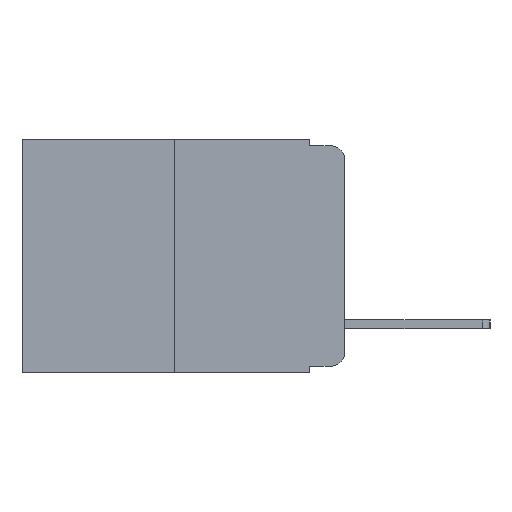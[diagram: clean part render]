
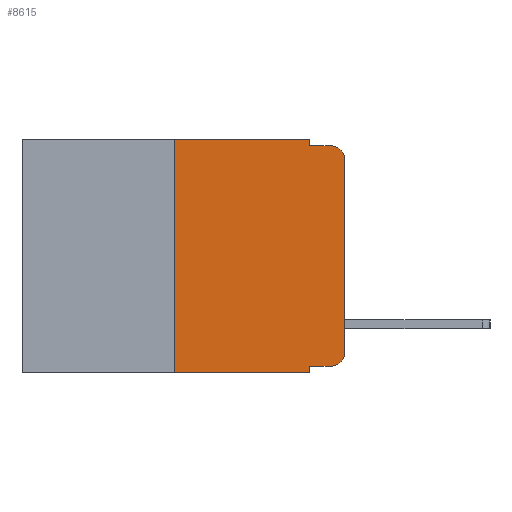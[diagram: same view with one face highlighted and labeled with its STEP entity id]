
A CAD part, left-side view. The second image highlights one B-rep face of the part: STEP entity #8615.
In plain terms, the highlighted planar face has unit normal (-1, 0, 0).
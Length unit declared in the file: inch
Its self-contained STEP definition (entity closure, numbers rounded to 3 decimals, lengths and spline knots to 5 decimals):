
#143 = FACE_OUTER_BOUND ( 'NONE', #7279, .T. ) ;
#237 = LINE ( 'NONE', #8047, #12402 ) ;
#459 = ORIENTED_EDGE ( 'NONE', *, *, #11915, .T. ) ;
#622 = CARTESIAN_POINT ( 'NONE',  ( 0., 0., -0.03 ) ) ;
#645 = PLANE ( 'NONE',  #2791 ) ;
#674 = ORIENTED_EDGE ( 'NONE', *, *, #12415, .T. ) ;
#821 = VECTOR ( 'NONE', #10563, 39.37008 ) ;
#980 = CIRCLE ( 'NONE', #7536, 0.02 ) ;
#990 = CARTESIAN_POINT ( 'NONE',  ( 0., 0.02, -0.03 ) ) ;
#1172 = CARTESIAN_POINT ( 'NONE',  ( 0., 0.25, 0. ) ) ;
#1273 = CARTESIAN_POINT ( 'NONE',  ( 0., 0.25, -0.343 ) ) ;
#1564 = VECTOR ( 'NONE', #3622, 39.37008 ) ;
#1577 = DIRECTION ( 'NONE',  ( 0., -1., 0. ) ) ;
#1594 = DIRECTION ( 'NONE',  ( 0., 0., -1. ) ) ;
#1650 = CARTESIAN_POINT ( 'NONE',  ( 0., 0.473, -0.343 ) ) ;
#1664 = VERTEX_POINT ( 'NONE', #1273 ) ;
#1936 = DIRECTION ( 'NONE',  ( 0., 0., -1. ) ) ;
#2309 = AXIS2_PLACEMENT_3D ( 'NONE', #3073, #9884, #4076 ) ;
#2432 = CARTESIAN_POINT ( 'NONE',  ( 0., 0.25, 0. ) ) ;
#2791 = AXIS2_PLACEMENT_3D ( 'NONE', #11223, #7389, #1594 ) ;
#2829 = VERTEX_POINT ( 'NONE', #8810 ) ;
#3045 = VECTOR ( 'NONE', #7934, 39.37008 ) ;
#3073 = CARTESIAN_POINT ( 'NONE',  ( 0., 0.02, -0.313 ) ) ;
#3076 = CARTESIAN_POINT ( 'NONE',  ( 0., 0., -0.313 ) ) ;
#3243 = EDGE_CURVE ( 'NONE', #12396, #8947, #980, .T. ) ;
#3322 = VECTOR ( 'NONE', #12444, 39.37008 ) ;
#3503 = CARTESIAN_POINT ( 'NONE',  ( 0., 0.051, -0.333 ) ) ;
#3551 = ORIENTED_EDGE ( 'NONE', *, *, #3653, .T. ) ;
#3622 = DIRECTION ( 'NONE',  ( 0., -1., 0. ) ) ;
#3653 = EDGE_CURVE ( 'NONE', #1664, #4661, #4457, .T. ) ;
#3947 = EDGE_CURVE ( 'NONE', #7925, #6077, #5672, .T. ) ;
#3960 = VECTOR ( 'NONE', #7903, 39.37008 ) ;
#4023 = EDGE_CURVE ( 'NONE', #6077, #8228, #237, .T. ) ;
#4049 = CARTESIAN_POINT ( 'NONE',  ( 0., 0.051, 0. ) ) ;
#4076 = DIRECTION ( 'NONE',  ( 0., 0., -1. ) ) ;
#4186 = DIRECTION ( 'NONE',  ( 0., 0., -1. ) ) ;
#4278 = ORIENTED_EDGE ( 'NONE', *, *, #11878, .F. ) ;
#4457 = LINE ( 'NONE', #1650, #1564 ) ;
#4657 = EDGE_CURVE ( 'NONE', #4885, #12396, #11209, .T. ) ;
#4661 = VERTEX_POINT ( 'NONE', #4732 ) ;
#4708 = VERTEX_POINT ( 'NONE', #4804 ) ;
#4732 = CARTESIAN_POINT ( 'NONE',  ( 0., 0.051, -0.343 ) ) ;
#4804 = CARTESIAN_POINT ( 'NONE',  ( 0., 0.02, -0.333 ) ) ;
#4885 = VERTEX_POINT ( 'NONE', #3076 ) ;
#4922 = ORIENTED_EDGE ( 'NONE', *, *, #11951, .F. ) ;
#5312 = ORIENTED_EDGE ( 'NONE', *, *, #4657, .T. ) ;
#5422 = ORIENTED_EDGE ( 'NONE', *, *, #3243, .T. ) ;
#5672 = LINE ( 'NONE', #8899, #3045 ) ;
#5780 = CARTESIAN_POINT ( 'NONE',  ( 0., 0.051, -0.01 ) ) ;
#5969 = LINE ( 'NONE', #1172, #3322 ) ;
#6006 = LINE ( 'NONE', #5780, #821 ) ;
#6077 = VERTEX_POINT ( 'NONE', #4049 ) ;
#6549 = LINE ( 'NONE', #11723, #3960 ) ;
#7279 = EDGE_LOOP ( 'NONE', ( #5312, #5422, #11512, #7449, #9998, #4922, #3551, #4278, #674, #459 ) ) ;
#7389 = DIRECTION ( 'NONE',  ( 1., 0., 0. ) ) ;
#7449 = ORIENTED_EDGE ( 'NONE', *, *, #4023, .F. ) ;
#7536 = AXIS2_PLACEMENT_3D ( 'NONE', #990, #7769, #1936 ) ;
#7769 = DIRECTION ( 'NONE',  ( -1., 0., 0. ) ) ;
#7903 = DIRECTION ( 'NONE',  ( 0., 0., -1. ) ) ;
#7925 = VERTEX_POINT ( 'NONE', #2432 ) ;
#7934 = DIRECTION ( 'NONE',  ( 0., -1., 0. ) ) ;
#8047 = CARTESIAN_POINT ( 'NONE',  ( 0., 0.051, 0. ) ) ;
#8228 = VERTEX_POINT ( 'NONE', #9648 ) ;
#8615 = ADVANCED_FACE ( 'NONE', ( #143 ), #645, .F. ) ;
#8810 = CARTESIAN_POINT ( 'NONE',  ( 0., 0.051, -0.333 ) ) ;
#8823 = CIRCLE ( 'NONE', #2309, 0.02 ) ;
#8899 = CARTESIAN_POINT ( 'NONE',  ( 0., 0.473, 0. ) ) ;
#8947 = VERTEX_POINT ( 'NONE', #9805 ) ;
#9648 = CARTESIAN_POINT ( 'NONE',  ( 0., 0.051, -0.01 ) ) ;
#9805 = CARTESIAN_POINT ( 'NONE',  ( 0., 0.02, -0.01 ) ) ;
#9884 = DIRECTION ( 'NONE',  ( -1., 0., 0. ) ) ;
#9998 = ORIENTED_EDGE ( 'NONE', *, *, #3947, .F. ) ;
#10033 = VECTOR ( 'NONE', #1577, 39.37008 ) ;
#10506 = CARTESIAN_POINT ( 'NONE',  ( 0., 0., 0. ) ) ;
#10563 = DIRECTION ( 'NONE',  ( 0., -1., 0. ) ) ;
#10576 = EDGE_CURVE ( 'NONE', #8228, #8947, #6006, .T. ) ;
#10922 = VECTOR ( 'NONE', #11462, 39.37008 ) ;
#11209 = LINE ( 'NONE', #10506, #10922 ) ;
#11214 = LINE ( 'NONE', #3503, #10033 ) ;
#11223 = CARTESIAN_POINT ( 'NONE',  ( 0., 0.473, 0. ) ) ;
#11462 = DIRECTION ( 'NONE',  ( 0., 0., 1. ) ) ;
#11512 = ORIENTED_EDGE ( 'NONE', *, *, #10576, .F. ) ;
#11723 = CARTESIAN_POINT ( 'NONE',  ( 0., 0.051, 0. ) ) ;
#11878 = EDGE_CURVE ( 'NONE', #2829, #4661, #6549, .T. ) ;
#11915 = EDGE_CURVE ( 'NONE', #4708, #4885, #8823, .T. ) ;
#11951 = EDGE_CURVE ( 'NONE', #1664, #7925, #5969, .T. ) ;
#12396 = VERTEX_POINT ( 'NONE', #622 ) ;
#12402 = VECTOR ( 'NONE', #4186, 39.37008 ) ;
#12415 = EDGE_CURVE ( 'NONE', #2829, #4708, #11214, .T. ) ;
#12444 = DIRECTION ( 'NONE',  ( 0., 0., 1. ) ) ;
